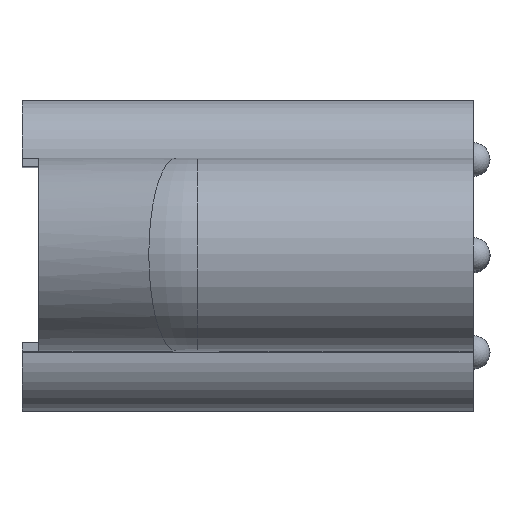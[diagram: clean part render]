
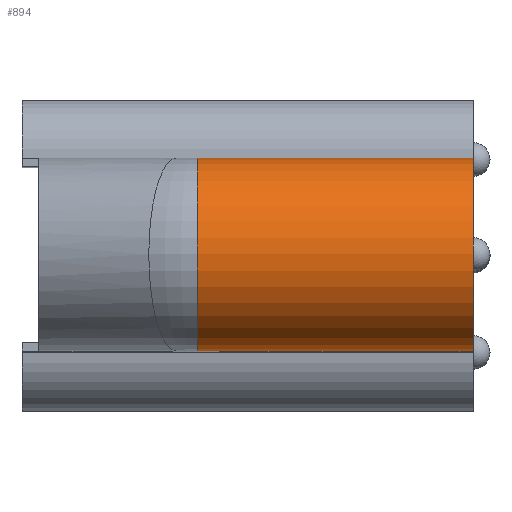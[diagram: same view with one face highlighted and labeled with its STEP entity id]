
A CAD part, top view. The second image highlights one B-rep face of the part: STEP entity #894.
In plain terms, the highlighted cylindrical face has radius 11.509 mm (diameter 23.019 mm), a partial arc.
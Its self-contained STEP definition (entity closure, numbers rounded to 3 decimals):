
#41 = DIRECTION ( 'NONE',  ( -1., 0., 0. ) ) ;
#84 = VECTOR ( 'NONE', #41, 1000. ) ;
#87 = CARTESIAN_POINT ( 'NONE',  ( 110.813, -25.532, 58.974 ) ) ;
#94 = LINE ( 'NONE', #87, #84 ) ;
#232 = EDGE_CURVE ( 'NONE', #1312, #954, #94, .T. ) ;
#335 = ORIENTED_EDGE ( 'NONE', *, *, #232, .F. ) ;
#340 = ORIENTED_EDGE ( 'NONE', *, *, #1889, .T. ) ;
#343 = ORIENTED_EDGE ( 'NONE', *, *, #2193, .F. ) ;
#347 = ORIENTED_EDGE ( 'NONE', *, *, #1695, .T. ) ;
#370 = VECTOR ( 'NONE', #1908, 1000. ) ;
#487 = LINE ( 'NONE', #1839, #370 ) ;
#505 = EDGE_LOOP ( 'NONE', ( #335, #340, #343, #347 ) ) ;
#651 = DIRECTION ( 'NONE',  ( 0., -1., 0. ) ) ;
#653 = DIRECTION ( 'NONE',  ( -1., 0., 0. ) ) ;
#655 = VERTEX_POINT ( 'NONE', #1970 ) ;
#656 = CARTESIAN_POINT ( 'NONE',  ( 8.61, -14.022, 58.974 ) ) ;
#894 = ADVANCED_FACE ( 'NONE', ( #1940 ), #1897, .T. ) ;
#920 = DIRECTION ( 'NONE',  ( 0., -1., 0. ) ) ;
#922 = DIRECTION ( 'NONE',  ( 1., 0., 0. ) ) ;
#929 = CARTESIAN_POINT ( 'NONE',  ( -24.311, -14.022, 58.974 ) ) ;
#954 = VERTEX_POINT ( 'NONE', #1683 ) ;
#1037 = CIRCLE ( 'NONE', #1202, 11.509 ) ;
#1115 = VERTEX_POINT ( 'NONE', #1617 ) ;
#1202 = AXIS2_PLACEMENT_3D ( 'NONE', #656, #653, #651 ) ;
#1207 = CIRCLE ( 'NONE', #1231, 11.509 ) ;
#1231 = AXIS2_PLACEMENT_3D ( 'NONE', #929, #922, #920 ) ;
#1312 = VERTEX_POINT ( 'NONE', #1375 ) ;
#1375 = CARTESIAN_POINT ( 'NONE',  ( 8.61, -25.532, 58.974 ) ) ;
#1528 = AXIS2_PLACEMENT_3D ( 'NONE', #1733, #1739, #1735 ) ;
#1617 = CARTESIAN_POINT ( 'NONE',  ( 8.61, -2.513, 58.974 ) ) ;
#1683 = CARTESIAN_POINT ( 'NONE',  ( -24.311, -25.532, 58.974 ) ) ;
#1695 = EDGE_CURVE ( 'NONE', #655, #954, #1207, .T. ) ;
#1733 = CARTESIAN_POINT ( 'NONE',  ( 12.729, -14.022, 58.974 ) ) ;
#1735 = DIRECTION ( 'NONE',  ( 0., -1., 0. ) ) ;
#1739 = DIRECTION ( 'NONE',  ( 1., 0., 0. ) ) ;
#1839 = CARTESIAN_POINT ( 'NONE',  ( 12.729, -2.513, 58.974 ) ) ;
#1889 = EDGE_CURVE ( 'NONE', #1312, #1115, #1037, .T. ) ;
#1897 = CYLINDRICAL_SURFACE ( 'NONE', #1528, 11.509 ) ;
#1908 = DIRECTION ( 'NONE',  ( 1., 0., 0. ) ) ;
#1940 = FACE_OUTER_BOUND ( 'NONE', #505, .T. ) ;
#1970 = CARTESIAN_POINT ( 'NONE',  ( -24.311, -2.513, 58.974 ) ) ;
#2193 = EDGE_CURVE ( 'NONE', #655, #1115, #487, .T. ) ;
